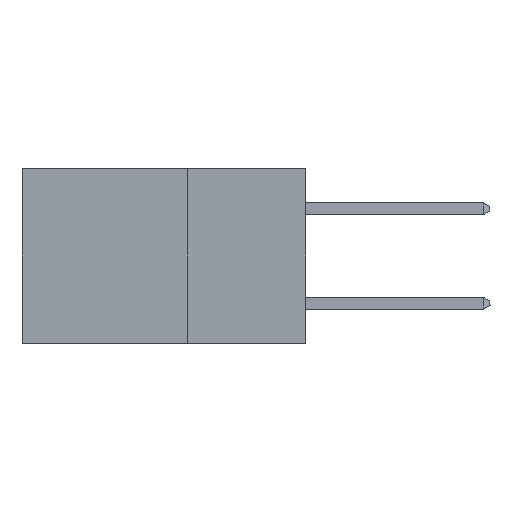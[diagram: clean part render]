
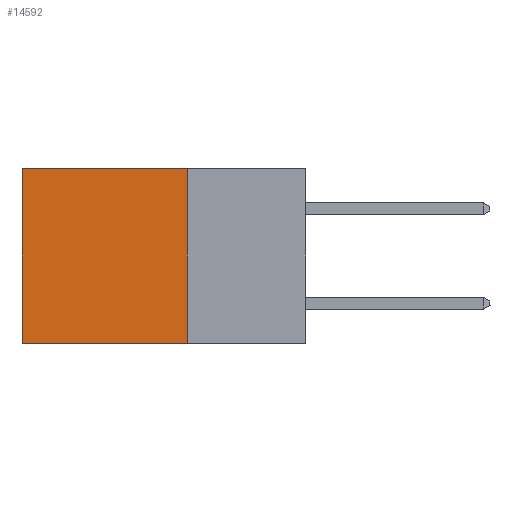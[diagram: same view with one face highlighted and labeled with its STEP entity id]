
A CAD part, left-side view. The second image highlights one B-rep face of the part: STEP entity #14592.
In plain terms, the highlighted planar face has unit normal (-1, 0, 0).
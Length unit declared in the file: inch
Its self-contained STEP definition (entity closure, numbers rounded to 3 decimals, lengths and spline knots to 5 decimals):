
#100 = AXIS2_PLACEMENT_3D ( 'NONE', #25288, #20776, #6852 ) ;
#575 = CARTESIAN_POINT ( 'NONE',  ( 0.298, 0.25, 0. ) ) ;
#688 = CARTESIAN_POINT ( 'NONE',  ( 0.298, 0.6, 0. ) ) ;
#3183 = ORIENTED_EDGE ( 'NONE', *, *, #7827, .F. ) ;
#3826 = LINE ( 'NONE', #29421, #21661 ) ;
#4460 = PLANE ( 'NONE',  #100 ) ;
#4719 = CARTESIAN_POINT ( 'NONE',  ( 0.298, 0.6, -0.37 ) ) ;
#6709 = EDGE_CURVE ( 'NONE', #16382, #25309, #27927, .T. ) ;
#6852 = DIRECTION ( 'NONE',  ( 0., 0., -1. ) ) ;
#7827 = EDGE_CURVE ( 'NONE', #8857, #16382, #23548, .T. ) ;
#8857 = VERTEX_POINT ( 'NONE', #23966 ) ;
#10071 = CARTESIAN_POINT ( 'NONE',  ( 0.298, 0.25, -0.37 ) ) ;
#10395 = EDGE_CURVE ( 'NONE', #8857, #23186, #28420, .T. ) ;
#14592 = ADVANCED_FACE ( 'NONE', ( #27475 ), #4460, .F. ) ;
#14773 = DIRECTION ( 'NONE',  ( 0., 1., 0. ) ) ;
#15509 = VECTOR ( 'NONE', #29468, 39.37008 ) ;
#15654 = CARTESIAN_POINT ( 'NONE',  ( 0.298, 0.25, -0.37 ) ) ;
#15732 = VECTOR ( 'NONE', #14773, 39.37008 ) ;
#16382 = VERTEX_POINT ( 'NONE', #15654 ) ;
#18686 = ORIENTED_EDGE ( 'NONE', *, *, #10395, .T. ) ;
#20719 = EDGE_CURVE ( 'NONE', #23186, #25309, #3826, .T. ) ;
#20776 = DIRECTION ( 'NONE',  ( 1., 0., 0. ) ) ;
#21576 = DIRECTION ( 'NONE',  ( 0., 0., -1. ) ) ;
#21661 = VECTOR ( 'NONE', #22637, 39.37008 ) ;
#22345 = EDGE_LOOP ( 'NONE', ( #22779, #25092, #3183, #18686 ) ) ;
#22637 = DIRECTION ( 'NONE',  ( 0., 0., -1. ) ) ;
#22779 = ORIENTED_EDGE ( 'NONE', *, *, #20719, .T. ) ;
#23186 = VERTEX_POINT ( 'NONE', #688 ) ;
#23548 = LINE ( 'NONE', #575, #28877 ) ;
#23966 = CARTESIAN_POINT ( 'NONE',  ( 0.298, 0.25, 0. ) ) ;
#25092 = ORIENTED_EDGE ( 'NONE', *, *, #6709, .F. ) ;
#25288 = CARTESIAN_POINT ( 'NONE',  ( 0.298, 0.25, 0. ) ) ;
#25309 = VERTEX_POINT ( 'NONE', #4719 ) ;
#27183 = CARTESIAN_POINT ( 'NONE',  ( 0.298, 0.25, 0. ) ) ;
#27475 = FACE_OUTER_BOUND ( 'NONE', #22345, .T. ) ;
#27927 = LINE ( 'NONE', #10071, #15732 ) ;
#28420 = LINE ( 'NONE', #27183, #15509 ) ;
#28877 = VECTOR ( 'NONE', #21576, 39.37008 ) ;
#29421 = CARTESIAN_POINT ( 'NONE',  ( 0.298, 0.6, 0. ) ) ;
#29468 = DIRECTION ( 'NONE',  ( 0., 1., 0. ) ) ;
